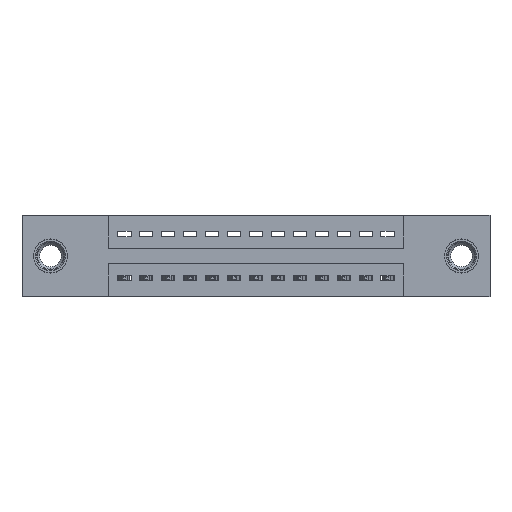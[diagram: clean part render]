
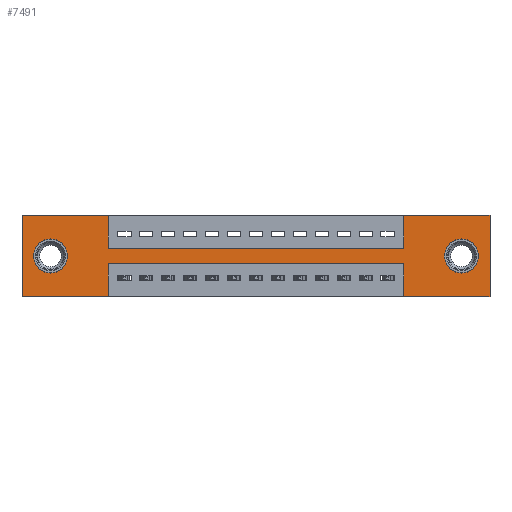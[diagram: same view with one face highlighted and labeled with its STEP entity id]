
A CAD part, front view. The second image highlights one B-rep face of the part: STEP entity #7491.
In plain terms, the highlighted planar face has unit normal (0, -1, 0).
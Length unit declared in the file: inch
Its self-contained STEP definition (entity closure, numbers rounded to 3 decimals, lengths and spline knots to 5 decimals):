
#27 = DIRECTION ( 'NONE',  ( 1., 0., 0. ) ) ;
#129 = VECTOR ( 'NONE', #14826, 39.37008 ) ;
#135 = AXIS2_PLACEMENT_3D ( 'NONE', #4522, #2297, #5565 ) ;
#153 = CARTESIAN_POINT ( 'NONE',  ( 1.7425, 0., -0.37 ) ) ;
#412 = DIRECTION ( 'NONE',  ( 0., 1., 0. ) ) ;
#557 = CARTESIAN_POINT ( 'NONE',  ( 0.13, 0., -0.107 ) ) ;
#607 = CARTESIAN_POINT ( 'NONE',  ( 0., 0., -0.37 ) ) ;
#629 = EDGE_CURVE ( 'NONE', #13917, #7589, #9883, .T. ) ;
#673 = LINE ( 'NONE', #13863, #11426 ) ;
#811 = EDGE_LOOP ( 'NONE', ( #2006, #4184 ) ) ;
#827 = EDGE_CURVE ( 'NONE', #10832, #1505, #6135, .T. ) ;
#1118 = VERTEX_POINT ( 'NONE', #14650 ) ;
#1505 = VERTEX_POINT ( 'NONE', #5685 ) ;
#1642 = EDGE_CURVE ( 'NONE', #1505, #5218, #5961, .T. ) ;
#1669 = VECTOR ( 'NONE', #5894, 39.37008 ) ;
#1721 = VERTEX_POINT ( 'NONE', #14416 ) ;
#2006 = ORIENTED_EDGE ( 'NONE', *, *, #14028, .T. ) ;
#2149 = DIRECTION ( 'NONE',  ( -1., 0., 0. ) ) ;
#2297 = DIRECTION ( 'NONE',  ( 0., 1., 0. ) ) ;
#2423 = DIRECTION ( 'NONE',  ( 0., 0., -1. ) ) ;
#2564 = CARTESIAN_POINT ( 'NONE',  ( 1.7425, 0., 0. ) ) ;
#2660 = VERTEX_POINT ( 'NONE', #5867 ) ;
#2872 = EDGE_LOOP ( 'NONE', ( #4203, #13260, #5361, #12708, #14033, #9472, #4593, #14339, #4627, #7181, #12675, #7658 ) ) ;
#2916 = CARTESIAN_POINT ( 'NONE',  ( 0.3925, 0., -0.15 ) ) ;
#2941 = CIRCLE ( 'NONE', #135, 0.078 ) ;
#3021 = EDGE_CURVE ( 'NONE', #5218, #12438, #11863, .T. ) ;
#3194 = DIRECTION ( 'NONE',  ( 0., 0., 1. ) ) ;
#3219 = LINE ( 'NONE', #5683, #129 ) ;
#3254 = VERTEX_POINT ( 'NONE', #13296 ) ;
#3438 = CARTESIAN_POINT ( 'NONE',  ( 1.7425, 0., -0.22 ) ) ;
#3610 = VERTEX_POINT ( 'NONE', #9957 ) ;
#3646 = LINE ( 'NONE', #9484, #11691 ) ;
#3879 = VERTEX_POINT ( 'NONE', #557 ) ;
#3925 = EDGE_CURVE ( 'NONE', #6498, #1721, #12013, .T. ) ;
#4184 = ORIENTED_EDGE ( 'NONE', *, *, #8427, .T. ) ;
#4203 = ORIENTED_EDGE ( 'NONE', *, *, #10586, .F. ) ;
#4343 = DIRECTION ( 'NONE',  ( 0., 1., 0. ) ) ;
#4522 = CARTESIAN_POINT ( 'NONE',  ( 2.005, 0., -0.185 ) ) ;
#4593 = ORIENTED_EDGE ( 'NONE', *, *, #1642, .F. ) ;
#4627 = ORIENTED_EDGE ( 'NONE', *, *, #11724, .F. ) ;
#5176 = CARTESIAN_POINT ( 'NONE',  ( 0., 0., 0. ) ) ;
#5218 = VERTEX_POINT ( 'NONE', #6928 ) ;
#5222 = DIRECTION ( 'NONE',  ( 1., 0., 0. ) ) ;
#5361 = ORIENTED_EDGE ( 'NONE', *, *, #629, .F. ) ;
#5497 = EDGE_CURVE ( 'NONE', #12438, #2660, #673, .T. ) ;
#5517 = AXIS2_PLACEMENT_3D ( 'NONE', #13151, #7633, #14369 ) ;
#5565 = DIRECTION ( 'NONE',  ( 0., 0., -1. ) ) ;
#5669 = AXIS2_PLACEMENT_3D ( 'NONE', #11954, #6433, #14447 ) ;
#5683 = CARTESIAN_POINT ( 'NONE',  ( 0., 0., 0. ) ) ;
#5685 = CARTESIAN_POINT ( 'NONE',  ( 1.7425, 0., -0.15 ) ) ;
#5851 = ORIENTED_EDGE ( 'NONE', *, *, #11687, .T. ) ;
#5867 = CARTESIAN_POINT ( 'NONE',  ( 2.135, 0., -0.37 ) ) ;
#5894 = DIRECTION ( 'NONE',  ( 0., 0., 1. ) ) ;
#5961 = LINE ( 'NONE', #2564, #8288 ) ;
#6135 = LINE ( 'NONE', #12194, #14602 ) ;
#6433 = DIRECTION ( 'NONE',  ( 0., 1., 0. ) ) ;
#6498 = VERTEX_POINT ( 'NONE', #7110 ) ;
#6718 = CIRCLE ( 'NONE', #14875, 0.078 ) ;
#6895 = EDGE_CURVE ( 'NONE', #3610, #12227, #10134, .T. ) ;
#6928 = CARTESIAN_POINT ( 'NONE',  ( 1.7425, 0., 0. ) ) ;
#6961 = DIRECTION ( 'NONE',  ( 0., 0., -1. ) ) ;
#7110 = CARTESIAN_POINT ( 'NONE',  ( 0.3925, 0., -0.37 ) ) ;
#7181 = ORIENTED_EDGE ( 'NONE', *, *, #6895, .F. ) ;
#7358 = CIRCLE ( 'NONE', #12597, 0.078 ) ;
#7491 = ADVANCED_FACE ( 'NONE', ( #13545, #11543, #14076 ), #12029, .T. ) ;
#7589 = VERTEX_POINT ( 'NONE', #3438 ) ;
#7633 = DIRECTION ( 'NONE',  ( 0., -1., 0. ) ) ;
#7658 = ORIENTED_EDGE ( 'NONE', *, *, #3925, .F. ) ;
#7889 = CARTESIAN_POINT ( 'NONE',  ( 0.13, 0., -0.185 ) ) ;
#8021 = CARTESIAN_POINT ( 'NONE',  ( 0., 0., 0. ) ) ;
#8214 = VERTEX_POINT ( 'NONE', #12690 ) ;
#8274 = CIRCLE ( 'NONE', #5669, 0.078 ) ;
#8288 = VECTOR ( 'NONE', #10892, 39.37008 ) ;
#8403 = EDGE_CURVE ( 'NONE', #2660, #13917, #8800, .T. ) ;
#8427 = EDGE_CURVE ( 'NONE', #3254, #3879, #7358, .T. ) ;
#8438 = VECTOR ( 'NONE', #2149, 39.37008 ) ;
#8614 = DIRECTION ( 'NONE',  ( -1., 0., 0. ) ) ;
#8626 = DIRECTION ( 'NONE',  ( 0., 0., -1. ) ) ;
#8698 = CARTESIAN_POINT ( 'NONE',  ( 2.135, 0., 0. ) ) ;
#8800 = LINE ( 'NONE', #9039, #8438 ) ;
#8823 = VECTOR ( 'NONE', #5222, 39.37008 ) ;
#9039 = CARTESIAN_POINT ( 'NONE',  ( 0., 0., -0.37 ) ) ;
#9472 = ORIENTED_EDGE ( 'NONE', *, *, #3021, .F. ) ;
#9484 = CARTESIAN_POINT ( 'NONE',  ( 0.3925, 0., -0.22 ) ) ;
#9786 = VECTOR ( 'NONE', #2423, 39.37008 ) ;
#9883 = LINE ( 'NONE', #153, #1669 ) ;
#9925 = LINE ( 'NONE', #13152, #10479 ) ;
#9957 = CARTESIAN_POINT ( 'NONE',  ( 0., 0., 0. ) ) ;
#10010 = EDGE_CURVE ( 'NONE', #1721, #3610, #3219, .T. ) ;
#10134 = LINE ( 'NONE', #8021, #11007 ) ;
#10361 = CARTESIAN_POINT ( 'NONE',  ( 0.3925, 0., -0.37 ) ) ;
#10479 = VECTOR ( 'NONE', #8626, 39.37008 ) ;
#10563 = VECTOR ( 'NONE', #8614, 39.37008 ) ;
#10586 = EDGE_CURVE ( 'NONE', #8214, #6498, #12845, .T. ) ;
#10673 = DIRECTION ( 'NONE',  ( -1., 0., 0. ) ) ;
#10715 = DIRECTION ( 'NONE',  ( 0., 0., -1. ) ) ;
#10832 = VERTEX_POINT ( 'NONE', #2916 ) ;
#10892 = DIRECTION ( 'NONE',  ( 0., 0., 1. ) ) ;
#11007 = VECTOR ( 'NONE', #27, 39.37008 ) ;
#11094 = ORIENTED_EDGE ( 'NONE', *, *, #13176, .T. ) ;
#11214 = CARTESIAN_POINT ( 'NONE',  ( 2.005, 0., -0.107 ) ) ;
#11426 = VECTOR ( 'NONE', #6961, 39.37008 ) ;
#11543 = FACE_BOUND ( 'NONE', #811, .T. ) ;
#11687 = EDGE_CURVE ( 'NONE', #13713, #1118, #6718, .T. ) ;
#11691 = VECTOR ( 'NONE', #10673, 39.37008 ) ;
#11715 = CARTESIAN_POINT ( 'NONE',  ( 1.7425, 0., -0.37 ) ) ;
#11724 = EDGE_CURVE ( 'NONE', #12227, #10832, #9925, .T. ) ;
#11863 = LINE ( 'NONE', #5176, #8823 ) ;
#11892 = EDGE_LOOP ( 'NONE', ( #5851, #11094 ) ) ;
#11954 = CARTESIAN_POINT ( 'NONE',  ( 0.13, 0., -0.185 ) ) ;
#12013 = LINE ( 'NONE', #607, #10563 ) ;
#12029 = PLANE ( 'NONE',  #5517 ) ;
#12194 = CARTESIAN_POINT ( 'NONE',  ( 0.3925, 0., -0.15 ) ) ;
#12227 = VERTEX_POINT ( 'NONE', #13988 ) ;
#12438 = VERTEX_POINT ( 'NONE', #8698 ) ;
#12597 = AXIS2_PLACEMENT_3D ( 'NONE', #7889, #4343, #3194 ) ;
#12675 = ORIENTED_EDGE ( 'NONE', *, *, #10010, .F. ) ;
#12690 = CARTESIAN_POINT ( 'NONE',  ( 0.3925, 0., -0.22 ) ) ;
#12708 = ORIENTED_EDGE ( 'NONE', *, *, #8403, .F. ) ;
#12845 = LINE ( 'NONE', #10361, #9786 ) ;
#13151 = CARTESIAN_POINT ( 'NONE',  ( 0., 0., -0.37 ) ) ;
#13152 = CARTESIAN_POINT ( 'NONE',  ( 0.3925, 0., 0. ) ) ;
#13176 = EDGE_CURVE ( 'NONE', #1118, #13713, #2941, .T. ) ;
#13260 = ORIENTED_EDGE ( 'NONE', *, *, #13587, .F. ) ;
#13296 = CARTESIAN_POINT ( 'NONE',  ( 0.13, 0., -0.263 ) ) ;
#13382 = DIRECTION ( 'NONE',  ( 1., 0., 0. ) ) ;
#13545 = FACE_BOUND ( 'NONE', #11892, .T. ) ;
#13587 = EDGE_CURVE ( 'NONE', #7589, #8214, #3646, .T. ) ;
#13713 = VERTEX_POINT ( 'NONE', #11214 ) ;
#13863 = CARTESIAN_POINT ( 'NONE',  ( 2.135, 0., 0. ) ) ;
#13917 = VERTEX_POINT ( 'NONE', #11715 ) ;
#13988 = CARTESIAN_POINT ( 'NONE',  ( 0.3925, 0., 0. ) ) ;
#14028 = EDGE_CURVE ( 'NONE', #3879, #3254, #8274, .T. ) ;
#14033 = ORIENTED_EDGE ( 'NONE', *, *, #5497, .F. ) ;
#14076 = FACE_OUTER_BOUND ( 'NONE', #2872, .T. ) ;
#14268 = CARTESIAN_POINT ( 'NONE',  ( 2.005, 0., -0.185 ) ) ;
#14339 = ORIENTED_EDGE ( 'NONE', *, *, #827, .F. ) ;
#14369 = DIRECTION ( 'NONE',  ( 0., 0., -1. ) ) ;
#14416 = CARTESIAN_POINT ( 'NONE',  ( 0., 0., -0.37 ) ) ;
#14447 = DIRECTION ( 'NONE',  ( 0., 0., 1. ) ) ;
#14602 = VECTOR ( 'NONE', #13382, 39.37008 ) ;
#14650 = CARTESIAN_POINT ( 'NONE',  ( 2.005, 0., -0.263 ) ) ;
#14826 = DIRECTION ( 'NONE',  ( 0., 0., 1. ) ) ;
#14875 = AXIS2_PLACEMENT_3D ( 'NONE', #14268, #412, #10715 ) ;
